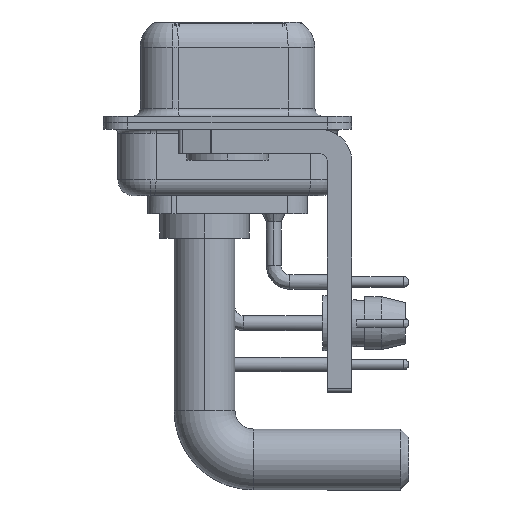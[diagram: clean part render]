
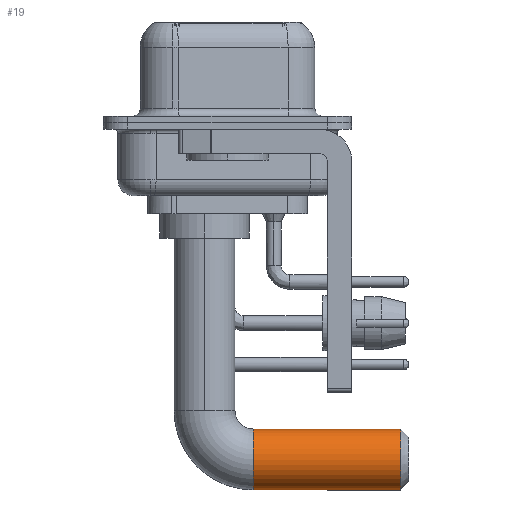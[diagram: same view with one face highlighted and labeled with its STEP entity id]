
A CAD part, left-side view. The second image highlights one B-rep face of the part: STEP entity #19.
In plain terms, the highlighted cylindrical face has radius 1.875 mm (diameter 3.75 mm), a partial arc.
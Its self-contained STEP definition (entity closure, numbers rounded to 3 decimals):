
#19 = ADVANCED_FACE ( 'NONE', ( #33674 ), #34194, .T. ) ;
#1159 = CARTESIAN_POINT ( 'NONE',  ( 0., -3., -11.755 ) ) ;
#1417 = CIRCLE ( 'NONE', #3649, 1.875 ) ;
#2765 = CARTESIAN_POINT ( 'NONE',  ( 0., -3., -11.755 ) ) ;
#3649 = AXIS2_PLACEMENT_3D ( 'NONE', #12870, #7048, #12529 ) ;
#3868 = CIRCLE ( 'NONE', #17956, 1.875 ) ;
#7048 = DIRECTION ( 'NONE',  ( 0., -1., 0. ) ) ;
#7190 = CARTESIAN_POINT ( 'NONE',  ( 0., -12.07, -11.755 ) ) ;
#8482 = VERTEX_POINT ( 'NONE', #19875 ) ;
#8566 = DIRECTION ( 'NONE',  ( 0., -1., 0. ) ) ;
#9807 = CARTESIAN_POINT ( 'NONE',  ( 0., -3., -15.505 ) ) ;
#10037 = EDGE_CURVE ( 'NONE', #8482, #25136, #3868, .T. ) ;
#10355 = AXIS2_PLACEMENT_3D ( 'NONE', #28696, #20764, #12641 ) ;
#12372 = VERTEX_POINT ( 'NONE', #2765 ) ;
#12529 = DIRECTION ( 'NONE',  ( -1., 0., 0. ) ) ;
#12641 = DIRECTION ( 'NONE',  ( 0., 0., -1. ) ) ;
#12870 = CARTESIAN_POINT ( 'NONE',  ( 0., -3., -13.63 ) ) ;
#13087 = ORIENTED_EDGE ( 'NONE', *, *, #24163, .F. ) ;
#17324 = LINE ( 'NONE', #27903, #34112 ) ;
#17470 = DIRECTION ( 'NONE',  ( 0., 0., -1. ) ) ;
#17956 = AXIS2_PLACEMENT_3D ( 'NONE', #20160, #30920, #17470 ) ;
#18938 = ORIENTED_EDGE ( 'NONE', *, *, #10037, .T. ) ;
#19785 = DIRECTION ( 'NONE',  ( 0., -1., 0. ) ) ;
#19875 = CARTESIAN_POINT ( 'NONE',  ( 0., -12.07, -15.505 ) ) ;
#20033 = LINE ( 'NONE', #1159, #29660 ) ;
#20160 = CARTESIAN_POINT ( 'NONE',  ( 0., -12.07, -13.63 ) ) ;
#20764 = DIRECTION ( 'NONE',  ( 0., -1., 0. ) ) ;
#22734 = EDGE_CURVE ( 'NONE', #27710, #8482, #17324, .T. ) ;
#24163 = EDGE_CURVE ( 'NONE', #12372, #25136, #20033, .T. ) ;
#25136 = VERTEX_POINT ( 'NONE', #7190 ) ;
#27710 = VERTEX_POINT ( 'NONE', #9807 ) ;
#27871 = EDGE_LOOP ( 'NONE', ( #13087, #33880, #34181, #18938 ) ) ;
#27903 = CARTESIAN_POINT ( 'NONE',  ( 0., -3., -15.505 ) ) ;
#28696 = CARTESIAN_POINT ( 'NONE',  ( 0., -3., -13.63 ) ) ;
#29660 = VECTOR ( 'NONE', #8566, 1000. ) ;
#30920 = DIRECTION ( 'NONE',  ( 0., 1., 0. ) ) ;
#31685 = EDGE_CURVE ( 'NONE', #12372, #27710, #1417, .T. ) ;
#33674 = FACE_OUTER_BOUND ( 'NONE', #27871, .T. ) ;
#33880 = ORIENTED_EDGE ( 'NONE', *, *, #31685, .T. ) ;
#34112 = VECTOR ( 'NONE', #19785, 1000. ) ;
#34181 = ORIENTED_EDGE ( 'NONE', *, *, #22734, .T. ) ;
#34194 = CYLINDRICAL_SURFACE ( 'NONE', #10355, 1.875 ) ;
